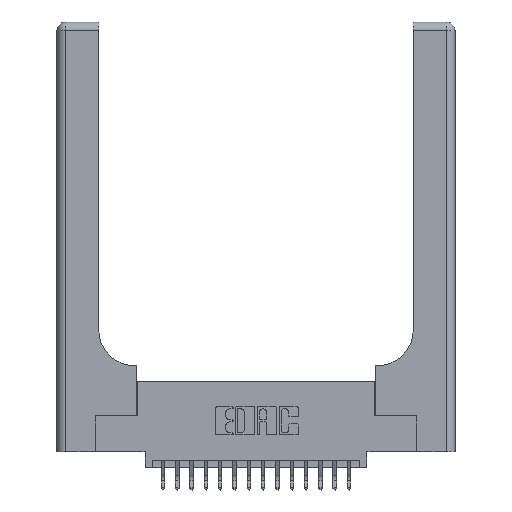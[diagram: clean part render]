
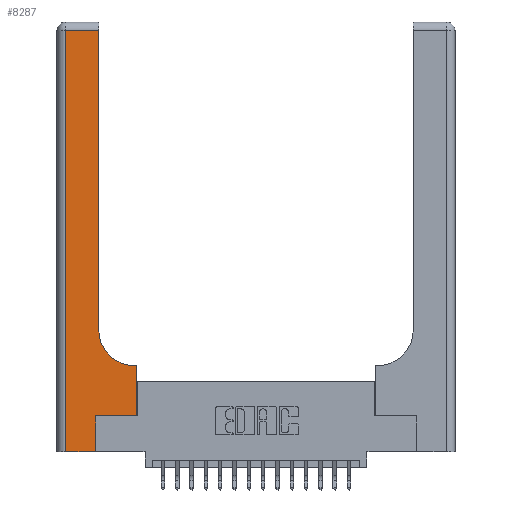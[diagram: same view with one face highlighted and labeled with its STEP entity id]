
A CAD part, top view. The second image highlights one B-rep face of the part: STEP entity #8287.
In plain terms, the highlighted planar face has unit normal (0, 0, 1).
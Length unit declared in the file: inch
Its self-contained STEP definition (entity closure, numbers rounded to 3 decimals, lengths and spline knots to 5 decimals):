
#267 = ORIENTED_EDGE ( 'NONE', *, *, #7901, .T. ) ;
#844 = EDGE_LOOP ( 'NONE', ( #11413, #14711, #1979, #10974, #9683, #267, #1789, #4277, #19123 ) ) ;
#1015 = VERTEX_POINT ( 'NONE', #9252 ) ;
#1054 = CARTESIAN_POINT ( 'NONE',  ( 0.269, 0., 0.37 ) ) ;
#1178 = DIRECTION ( 'NONE',  ( -1., 0., 0. ) ) ;
#1789 = ORIENTED_EDGE ( 'NONE', *, *, #14972, .T. ) ;
#1979 = ORIENTED_EDGE ( 'NONE', *, *, #18242, .T. ) ;
#2010 = LINE ( 'NONE', #9990, #6306 ) ;
#2506 = CARTESIAN_POINT ( 'NONE',  ( 0.2915, 2.94, 0.37 ) ) ;
#2546 = VECTOR ( 'NONE', #16316, 39.37008 ) ;
#2748 = VECTOR ( 'NONE', #17689, 39.37008 ) ;
#3065 = VECTOR ( 'NONE', #7144, 39.37008 ) ;
#3171 = DIRECTION ( 'NONE',  ( 0., 0., -1. ) ) ;
#3294 = LINE ( 'NONE', #13868, #11735 ) ;
#3626 = VERTEX_POINT ( 'NONE', #11240 ) ;
#3927 = VERTEX_POINT ( 'NONE', #1054 ) ;
#4169 = VECTOR ( 'NONE', #8956, 39.37008 ) ;
#4217 = VERTEX_POINT ( 'NONE', #11285 ) ;
#4277 = ORIENTED_EDGE ( 'NONE', *, *, #12406, .T. ) ;
#4454 = DIRECTION ( 'NONE',  ( 0., 1., 0. ) ) ;
#5520 = CARTESIAN_POINT ( 'NONE',  ( 0., 0., 0.37 ) ) ;
#6306 = VECTOR ( 'NONE', #9628, 39.37008 ) ;
#6604 = EDGE_CURVE ( 'NONE', #16098, #3626, #15110, .T. ) ;
#7144 = DIRECTION ( 'NONE',  ( 1., 0., 0. ) ) ;
#7379 = CARTESIAN_POINT ( 'NONE',  ( 0.2915, 3., 0.37 ) ) ;
#7691 = CIRCLE ( 'NONE', #9885, 0.25 ) ;
#7901 = EDGE_CURVE ( 'NONE', #9126, #4217, #10741, .T. ) ;
#8287 = ADVANCED_FACE ( 'NONE', ( #16264 ), #20270, .F. ) ;
#8511 = CARTESIAN_POINT ( 'NONE',  ( 0.269, 0.25, 0.37 ) ) ;
#8649 = VECTOR ( 'NONE', #16442, 39.37008 ) ;
#8868 = VERTEX_POINT ( 'NONE', #9753 ) ;
#8906 = VERTEX_POINT ( 'NONE', #11348 ) ;
#8956 = DIRECTION ( 'NONE',  ( 0., 1., 0. ) ) ;
#9126 = VERTEX_POINT ( 'NONE', #13425 ) ;
#9130 = LINE ( 'NONE', #14885, #8649 ) ;
#9252 = CARTESIAN_POINT ( 'NONE',  ( 0.5415, 0.6, 0.37 ) ) ;
#9272 = DIRECTION ( 'NONE',  ( 0., 0., -1. ) ) ;
#9628 = DIRECTION ( 'NONE',  ( 0., 1., 0. ) ) ;
#9683 = ORIENTED_EDGE ( 'NONE', *, *, #19223, .T. ) ;
#9753 = CARTESIAN_POINT ( 'NONE',  ( 0.5585, 0.6, 0.37 ) ) ;
#9885 = AXIS2_PLACEMENT_3D ( 'NONE', #18468, #9272, #19997 ) ;
#9990 = CARTESIAN_POINT ( 'NONE',  ( 0.5585, 0.25, 0.37 ) ) ;
#10741 = LINE ( 'NONE', #8511, #2748 ) ;
#10856 = LINE ( 'NONE', #19916, #14451 ) ;
#10974 = ORIENTED_EDGE ( 'NONE', *, *, #13495, .T. ) ;
#11240 = CARTESIAN_POINT ( 'NONE',  ( 0.06, 2.94, 0.37 ) ) ;
#11285 = CARTESIAN_POINT ( 'NONE',  ( 0.5585, 0.25, 0.37 ) ) ;
#11348 = CARTESIAN_POINT ( 'NONE',  ( 0.2915, 0.85, 0.37 ) ) ;
#11413 = ORIENTED_EDGE ( 'NONE', *, *, #11582, .T. ) ;
#11582 = EDGE_CURVE ( 'NONE', #8906, #16098, #16657, .T. ) ;
#11735 = VECTOR ( 'NONE', #4454, 39.37008 ) ;
#12406 = EDGE_CURVE ( 'NONE', #8868, #1015, #10856, .T. ) ;
#12659 = CARTESIAN_POINT ( 'NONE',  ( 0., 3., 0.37 ) ) ;
#13425 = CARTESIAN_POINT ( 'NONE',  ( 0.269, 0.25, 0.37 ) ) ;
#13495 = EDGE_CURVE ( 'NONE', #14540, #3927, #19668, .T. ) ;
#13868 = CARTESIAN_POINT ( 'NONE',  ( 0.269, 0., 0.37 ) ) ;
#14198 = DIRECTION ( 'NONE',  ( -1., 0., 0. ) ) ;
#14451 = VECTOR ( 'NONE', #1178, 39.37008 ) ;
#14540 = VERTEX_POINT ( 'NONE', #14622 ) ;
#14622 = CARTESIAN_POINT ( 'NONE',  ( 0.06, 0., 0.37 ) ) ;
#14711 = ORIENTED_EDGE ( 'NONE', *, *, #6604, .T. ) ;
#14761 = CARTESIAN_POINT ( 'NONE',  ( 0., 2.94, 0.37 ) ) ;
#14885 = CARTESIAN_POINT ( 'NONE',  ( 0.06, 3., 0.37 ) ) ;
#14972 = EDGE_CURVE ( 'NONE', #4217, #8868, #2010, .T. ) ;
#15110 = LINE ( 'NONE', #14761, #2546 ) ;
#16098 = VERTEX_POINT ( 'NONE', #2506 ) ;
#16264 = FACE_OUTER_BOUND ( 'NONE', #844, .T. ) ;
#16316 = DIRECTION ( 'NONE',  ( -1., 0., 0. ) ) ;
#16442 = DIRECTION ( 'NONE',  ( 0., -1., 0. ) ) ;
#16657 = LINE ( 'NONE', #7379, #4169 ) ;
#17333 = EDGE_CURVE ( 'NONE', #1015, #8906, #7691, .T. ) ;
#17689 = DIRECTION ( 'NONE',  ( 1., 0., 0. ) ) ;
#17862 = AXIS2_PLACEMENT_3D ( 'NONE', #12659, #3171, #14198 ) ;
#18242 = EDGE_CURVE ( 'NONE', #3626, #14540, #9130, .T. ) ;
#18468 = CARTESIAN_POINT ( 'NONE',  ( 0.5415, 0.85, 0.37 ) ) ;
#19123 = ORIENTED_EDGE ( 'NONE', *, *, #17333, .T. ) ;
#19223 = EDGE_CURVE ( 'NONE', #3927, #9126, #3294, .T. ) ;
#19668 = LINE ( 'NONE', #5520, #3065 ) ;
#19916 = CARTESIAN_POINT ( 'NONE',  ( 0.2915, 0.6, 0.37 ) ) ;
#19997 = DIRECTION ( 'NONE',  ( 1., 0., 0. ) ) ;
#20270 = PLANE ( 'NONE',  #17862 ) ;
